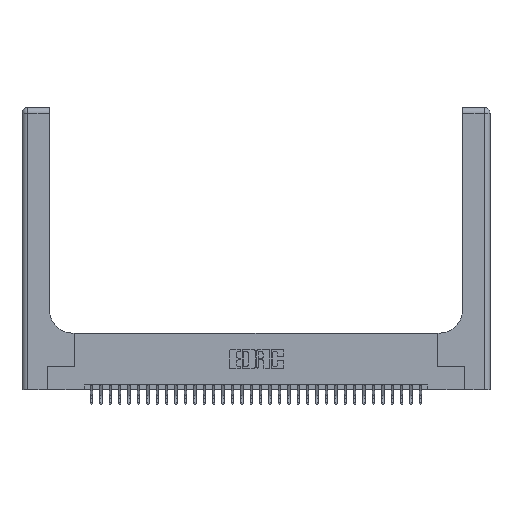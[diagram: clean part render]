
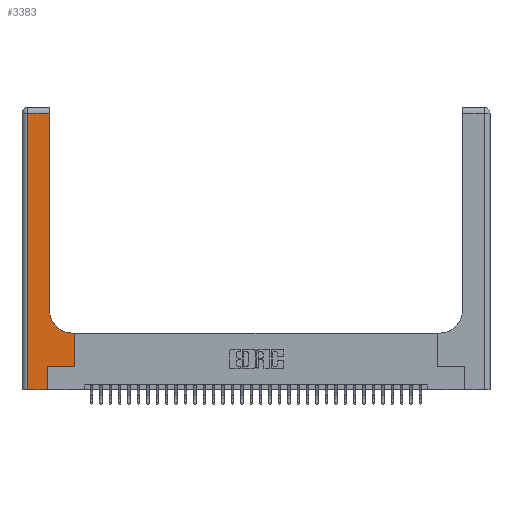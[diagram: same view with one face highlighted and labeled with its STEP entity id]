
A CAD part, top view. The second image highlights one B-rep face of the part: STEP entity #3383.
In plain terms, the highlighted planar face has unit normal (0, 0, 1).
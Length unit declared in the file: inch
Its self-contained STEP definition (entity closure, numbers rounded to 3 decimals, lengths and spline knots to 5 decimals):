
#1211 = DIRECTION ( 'NONE',  ( -1., 0., 0. ) ) ;
#2167 = PLANE ( 'NONE',  #18368 ) ;
#2278 = DIRECTION ( 'NONE',  ( -1., 0., 0. ) ) ;
#2899 = EDGE_CURVE ( 'NONE', #24472, #25176, #11220, .T. ) ;
#3090 = ORIENTED_EDGE ( 'NONE', *, *, #6974, .T. ) ;
#3146 = CARTESIAN_POINT ( 'NONE',  ( 0., 0., 0.37 ) ) ;
#3158 = VERTEX_POINT ( 'NONE', #17492 ) ;
#3199 = DIRECTION ( 'NONE',  ( 0., 1., 0. ) ) ;
#3383 = ADVANCED_FACE ( 'NONE', ( #12038 ), #2167, .F. ) ;
#3581 = CARTESIAN_POINT ( 'NONE',  ( 0.269, 0.25, 0.37 ) ) ;
#3952 = CARTESIAN_POINT ( 'NONE',  ( 0.2915, 0.6, 0.37 ) ) ;
#4110 = VECTOR ( 'NONE', #32415, 39.37008 ) ;
#4591 = VERTEX_POINT ( 'NONE', #12019 ) ;
#4682 = DIRECTION ( 'NONE',  ( 0., 1., 0. ) ) ;
#5052 = EDGE_CURVE ( 'NONE', #25217, #24472, #11482, .T. ) ;
#6081 = ORIENTED_EDGE ( 'NONE', *, *, #11926, .T. ) ;
#6448 = VECTOR ( 'NONE', #16416, 39.37008 ) ;
#6957 = AXIS2_PLACEMENT_3D ( 'NONE', #23348, #7387, #26011 ) ;
#6974 = EDGE_CURVE ( 'NONE', #32968, #4591, #11343, .T. ) ;
#7387 = DIRECTION ( 'NONE',  ( 0., 0., -1. ) ) ;
#8472 = VECTOR ( 'NONE', #1211, 39.37008 ) ;
#8668 = LINE ( 'NONE', #32398, #30621 ) ;
#9512 = CARTESIAN_POINT ( 'NONE',  ( 0.2915, 2.94, 0.37 ) ) ;
#10350 = ORIENTED_EDGE ( 'NONE', *, *, #20487, .T. ) ;
#11077 = CARTESIAN_POINT ( 'NONE',  ( 0.269, 0.25, 0.37 ) ) ;
#11220 = LINE ( 'NONE', #3146, #32270 ) ;
#11343 = LINE ( 'NONE', #29799, #4110 ) ;
#11482 = LINE ( 'NONE', #21719, #25557 ) ;
#11564 = CARTESIAN_POINT ( 'NONE',  ( 0.06, 2.94, 0.37 ) ) ;
#11926 = EDGE_CURVE ( 'NONE', #31616, #25217, #27079, .T. ) ;
#12019 = CARTESIAN_POINT ( 'NONE',  ( 0.5585, 0.6, 0.37 ) ) ;
#12038 = FACE_OUTER_BOUND ( 'NONE', #20379, .T. ) ;
#12997 = VECTOR ( 'NONE', #33237, 39.37008 ) ;
#13277 = VERTEX_POINT ( 'NONE', #21197 ) ;
#13991 = CARTESIAN_POINT ( 'NONE',  ( 0.269, 0., 0.37 ) ) ;
#14917 = ORIENTED_EDGE ( 'NONE', *, *, #2899, .T. ) ;
#15746 = CARTESIAN_POINT ( 'NONE',  ( 0., 3., 0.37 ) ) ;
#16416 = DIRECTION ( 'NONE',  ( 1., 0., 0. ) ) ;
#17492 = CARTESIAN_POINT ( 'NONE',  ( 0.2915, 0.85, 0.37 ) ) ;
#18368 = AXIS2_PLACEMENT_3D ( 'NONE', #15746, #18389, #2278 ) ;
#18389 = DIRECTION ( 'NONE',  ( 0., 0., -1. ) ) ;
#19236 = DIRECTION ( 'NONE',  ( 1., 0., 0. ) ) ;
#20379 = EDGE_LOOP ( 'NONE', ( #25680, #6081, #27321, #14917, #28968, #30605, #3090, #10350, #26102 ) ) ;
#20487 = EDGE_CURVE ( 'NONE', #4591, #13277, #22640, .T. ) ;
#20659 = LINE ( 'NONE', #11077, #6448 ) ;
#21197 = CARTESIAN_POINT ( 'NONE',  ( 0.5415, 0.6, 0.37 ) ) ;
#21719 = CARTESIAN_POINT ( 'NONE',  ( 0.06, 3., 0.37 ) ) ;
#22640 = LINE ( 'NONE', #3952, #8472 ) ;
#23348 = CARTESIAN_POINT ( 'NONE',  ( 0.5415, 0.85, 0.37 ) ) ;
#23443 = VECTOR ( 'NONE', #4682, 39.37008 ) ;
#24447 = CARTESIAN_POINT ( 'NONE',  ( 0.06, 0., 0.37 ) ) ;
#24472 = VERTEX_POINT ( 'NONE', #24447 ) ;
#25176 = VERTEX_POINT ( 'NONE', #13991 ) ;
#25217 = VERTEX_POINT ( 'NONE', #11564 ) ;
#25260 = VERTEX_POINT ( 'NONE', #3581 ) ;
#25557 = VECTOR ( 'NONE', #29646, 39.37008 ) ;
#25680 = ORIENTED_EDGE ( 'NONE', *, *, #34441, .T. ) ;
#25725 = CIRCLE ( 'NONE', #6957, 0.25 ) ;
#26011 = DIRECTION ( 'NONE',  ( 1., 0., 0. ) ) ;
#26102 = ORIENTED_EDGE ( 'NONE', *, *, #34143, .T. ) ;
#27079 = LINE ( 'NONE', #30641, #12997 ) ;
#27321 = ORIENTED_EDGE ( 'NONE', *, *, #5052, .T. ) ;
#28968 = ORIENTED_EDGE ( 'NONE', *, *, #30576, .T. ) ;
#29383 = EDGE_CURVE ( 'NONE', #25260, #32968, #20659, .T. ) ;
#29646 = DIRECTION ( 'NONE',  ( 0., -1., 0. ) ) ;
#29799 = CARTESIAN_POINT ( 'NONE',  ( 0.5585, 0.25, 0.37 ) ) ;
#30440 = LINE ( 'NONE', #31293, #23443 ) ;
#30576 = EDGE_CURVE ( 'NONE', #25176, #25260, #30440, .T. ) ;
#30605 = ORIENTED_EDGE ( 'NONE', *, *, #29383, .T. ) ;
#30621 = VECTOR ( 'NONE', #3199, 39.37008 ) ;
#30641 = CARTESIAN_POINT ( 'NONE',  ( 0., 2.94, 0.37 ) ) ;
#31293 = CARTESIAN_POINT ( 'NONE',  ( 0.269, 0., 0.37 ) ) ;
#31616 = VERTEX_POINT ( 'NONE', #9512 ) ;
#32270 = VECTOR ( 'NONE', #19236, 39.37008 ) ;
#32398 = CARTESIAN_POINT ( 'NONE',  ( 0.2915, 3., 0.37 ) ) ;
#32415 = DIRECTION ( 'NONE',  ( 0., 1., 0. ) ) ;
#32968 = VERTEX_POINT ( 'NONE', #34070 ) ;
#33237 = DIRECTION ( 'NONE',  ( -1., 0., 0. ) ) ;
#34070 = CARTESIAN_POINT ( 'NONE',  ( 0.5585, 0.25, 0.37 ) ) ;
#34143 = EDGE_CURVE ( 'NONE', #13277, #3158, #25725, .T. ) ;
#34441 = EDGE_CURVE ( 'NONE', #3158, #31616, #8668, .T. ) ;
